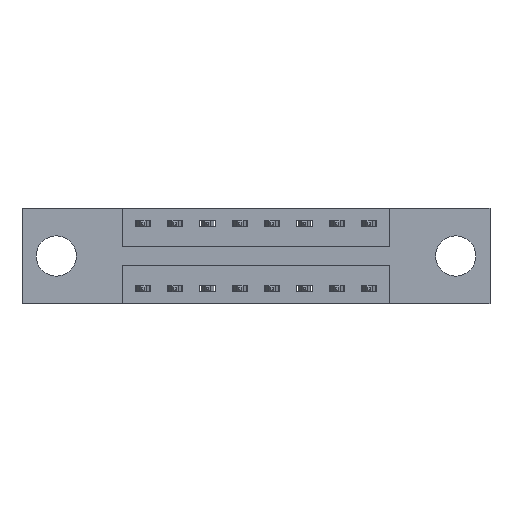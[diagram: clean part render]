
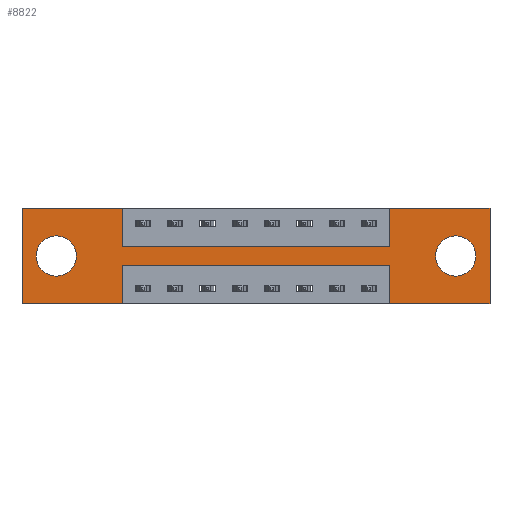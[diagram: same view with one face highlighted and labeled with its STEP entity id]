
A CAD part, front view. The second image highlights one B-rep face of the part: STEP entity #8822.
In plain terms, the highlighted planar face has unit normal (0, -1, 0).
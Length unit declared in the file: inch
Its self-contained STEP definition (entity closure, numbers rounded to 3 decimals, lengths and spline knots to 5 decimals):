
#18 = CIRCLE ( 'NONE', #1250, 0.078 ) ;
#73 = CARTESIAN_POINT ( 'NONE',  ( 0., 0., 0. ) ) ;
#162 = CARTESIAN_POINT ( 'NONE',  ( 0., 0., 0. ) ) ;
#163 = CARTESIAN_POINT ( 'NONE',  ( 1.6775, 0., -0.185 ) ) ;
#220 = CARTESIAN_POINT ( 'NONE',  ( 1.6775, 0., -0.263 ) ) ;
#240 = EDGE_CURVE ( 'NONE', #2358, #2981, #966, .T. ) ;
#244 = ORIENTED_EDGE ( 'NONE', *, *, #4521, .T. ) ;
#248 = VECTOR ( 'NONE', #5914, 39.37008 ) ;
#287 = CARTESIAN_POINT ( 'NONE',  ( 0., 0., -0.37 ) ) ;
#344 = DIRECTION ( 'NONE',  ( -1., 0., 0. ) ) ;
#372 = ORIENTED_EDGE ( 'NONE', *, *, #9281, .T. ) ;
#377 = VECTOR ( 'NONE', #1443, 39.37008 ) ;
#523 = CARTESIAN_POINT ( 'NONE',  ( 0.3875, 0., -0.15 ) ) ;
#602 = VECTOR ( 'NONE', #3147, 39.37008 ) ;
#604 = LINE ( 'NONE', #2105, #8022 ) ;
#612 = EDGE_CURVE ( 'NONE', #4456, #1969, #2550, .T. ) ;
#658 = EDGE_CURVE ( 'NONE', #5437, #5779, #6012, .T. ) ;
#760 = CARTESIAN_POINT ( 'NONE',  ( 0., 0., 0. ) ) ;
#766 = ORIENTED_EDGE ( 'NONE', *, *, #9006, .T. ) ;
#806 = ORIENTED_EDGE ( 'NONE', *, *, #4437, .F. ) ;
#897 = VERTEX_POINT ( 'NONE', #5946 ) ;
#966 = LINE ( 'NONE', #3966, #8792 ) ;
#1250 = AXIS2_PLACEMENT_3D ( 'NONE', #4259, #5805, #4326 ) ;
#1253 = VERTEX_POINT ( 'NONE', #4018 ) ;
#1443 = DIRECTION ( 'NONE',  ( 0., 0., -1. ) ) ;
#1598 = CIRCLE ( 'NONE', #2481, 0.078 ) ;
#1659 = ORIENTED_EDGE ( 'NONE', *, *, #9187, .F. ) ;
#1688 = DIRECTION ( 'NONE',  ( 0., 1., 0. ) ) ;
#1774 = ORIENTED_EDGE ( 'NONE', *, *, #240, .F. ) ;
#1795 = CARTESIAN_POINT ( 'NONE',  ( 0.1325, 0., -0.185 ) ) ;
#1802 = VECTOR ( 'NONE', #2873, 39.37008 ) ;
#1834 = LINE ( 'NONE', #760, #5275 ) ;
#1969 = VERTEX_POINT ( 'NONE', #3968 ) ;
#2040 = CARTESIAN_POINT ( 'NONE',  ( 1.4225, 0., -0.22 ) ) ;
#2066 = FACE_BOUND ( 'NONE', #4221, .T. ) ;
#2105 = CARTESIAN_POINT ( 'NONE',  ( 0., 0., 0. ) ) ;
#2180 = FACE_OUTER_BOUND ( 'NONE', #2342, .T. ) ;
#2183 = CIRCLE ( 'NONE', #5569, 0.078 ) ;
#2309 = FACE_BOUND ( 'NONE', #3071, .T. ) ;
#2311 = VECTOR ( 'NONE', #5316, 39.37008 ) ;
#2342 = EDGE_LOOP ( 'NONE', ( #7362, #7193, #8394, #806, #4942, #7039, #1659, #1774, #8101, #3868, #5143, #7452 ) ) ;
#2358 = VERTEX_POINT ( 'NONE', #523 ) ;
#2362 = VERTEX_POINT ( 'NONE', #7970 ) ;
#2425 = DIRECTION ( 'NONE',  ( 0., -1., 0. ) ) ;
#2481 = AXIS2_PLACEMENT_3D ( 'NONE', #1795, #7072, #8713 ) ;
#2550 = LINE ( 'NONE', #162, #602 ) ;
#2579 = CARTESIAN_POINT ( 'NONE',  ( 0.3875, 0., -0.22 ) ) ;
#2589 = CARTESIAN_POINT ( 'NONE',  ( 0.3875, 0., -0.37 ) ) ;
#2873 = DIRECTION ( 'NONE',  ( -1., 0., 0. ) ) ;
#2916 = EDGE_CURVE ( 'NONE', #5779, #5621, #9279, .T. ) ;
#2950 = VECTOR ( 'NONE', #7378, 39.37008 ) ;
#2981 = VERTEX_POINT ( 'NONE', #9341 ) ;
#2998 = CARTESIAN_POINT ( 'NONE',  ( 1.4225, 0., 0. ) ) ;
#3021 = EDGE_CURVE ( 'NONE', #9406, #4456, #1834, .T. ) ;
#3071 = EDGE_LOOP ( 'NONE', ( #3728, #766 ) ) ;
#3147 = DIRECTION ( 'NONE',  ( 1., 0., 0. ) ) ;
#3158 = DIRECTION ( 'NONE',  ( 0., 1., 0. ) ) ;
#3473 = VECTOR ( 'NONE', #344, 39.37008 ) ;
#3620 = CARTESIAN_POINT ( 'NONE',  ( 0.3875, 0., 0. ) ) ;
#3626 = LINE ( 'NONE', #3620, #377 ) ;
#3728 = ORIENTED_EDGE ( 'NONE', *, *, #3836, .T. ) ;
#3789 = LINE ( 'NONE', #7937, #1802 ) ;
#3836 = EDGE_CURVE ( 'NONE', #2362, #1253, #1598, .T. ) ;
#3864 = LINE ( 'NONE', #5879, #248 ) ;
#3868 = ORIENTED_EDGE ( 'NONE', *, *, #612, .F. ) ;
#3966 = CARTESIAN_POINT ( 'NONE',  ( 0.3875, 0., -0.15 ) ) ;
#3968 = CARTESIAN_POINT ( 'NONE',  ( 0.3875, 0., 0. ) ) ;
#3978 = CARTESIAN_POINT ( 'NONE',  ( 0.3875, 0., -0.37 ) ) ;
#4018 = CARTESIAN_POINT ( 'NONE',  ( 0.1325, 0., -0.263 ) ) ;
#4209 = VECTOR ( 'NONE', #5524, 39.37008 ) ;
#4221 = EDGE_LOOP ( 'NONE', ( #244, #372 ) ) ;
#4259 = CARTESIAN_POINT ( 'NONE',  ( 0.1325, 0., -0.185 ) ) ;
#4326 = DIRECTION ( 'NONE',  ( 0., 0., 1. ) ) ;
#4357 = CARTESIAN_POINT ( 'NONE',  ( 1.6775, 0., -0.107 ) ) ;
#4431 = LINE ( 'NONE', #5045, #2950 ) ;
#4437 = EDGE_CURVE ( 'NONE', #897, #6561, #3864, .T. ) ;
#4456 = VERTEX_POINT ( 'NONE', #73 ) ;
#4521 = EDGE_CURVE ( 'NONE', #7868, #5977, #8732, .T. ) ;
#4560 = VECTOR ( 'NONE', #6499, 39.37008 ) ;
#4563 = AXIS2_PLACEMENT_3D ( 'NONE', #287, #2425, #6246 ) ;
#4712 = CARTESIAN_POINT ( 'NONE',  ( 1.81, 0., 0. ) ) ;
#4804 = CARTESIAN_POINT ( 'NONE',  ( 1.4225, 0., 0. ) ) ;
#4942 = ORIENTED_EDGE ( 'NONE', *, *, #5248, .F. ) ;
#5045 = CARTESIAN_POINT ( 'NONE',  ( 1.4225, 0., -0.37 ) ) ;
#5143 = ORIENTED_EDGE ( 'NONE', *, *, #3021, .F. ) ;
#5198 = DIRECTION ( 'NONE',  ( 1., 0., 0. ) ) ;
#5248 = EDGE_CURVE ( 'NONE', #7309, #897, #6613, .T. ) ;
#5275 = VECTOR ( 'NONE', #7059, 39.37008 ) ;
#5316 = DIRECTION ( 'NONE',  ( 0., 0., 1. ) ) ;
#5411 = VERTEX_POINT ( 'NONE', #4804 ) ;
#5412 = CARTESIAN_POINT ( 'NONE',  ( 0.3875, 0., -0.22 ) ) ;
#5437 = VERTEX_POINT ( 'NONE', #2040 ) ;
#5457 = DIRECTION ( 'NONE',  ( 0., 0., -1. ) ) ;
#5524 = DIRECTION ( 'NONE',  ( 0., 0., -1. ) ) ;
#5569 = AXIS2_PLACEMENT_3D ( 'NONE', #163, #3158, #5457 ) ;
#5621 = VERTEX_POINT ( 'NONE', #2589 ) ;
#5779 = VERTEX_POINT ( 'NONE', #2579 ) ;
#5805 = DIRECTION ( 'NONE',  ( 0., 1., 0. ) ) ;
#5879 = CARTESIAN_POINT ( 'NONE',  ( 0., 0., -0.37 ) ) ;
#5914 = DIRECTION ( 'NONE',  ( -1., 0., 0. ) ) ;
#5946 = CARTESIAN_POINT ( 'NONE',  ( 1.81, 0., -0.37 ) ) ;
#5977 = VERTEX_POINT ( 'NONE', #220 ) ;
#6012 = LINE ( 'NONE', #5412, #3473 ) ;
#6090 = EDGE_CURVE ( 'NONE', #1969, #2358, #3626, .T. ) ;
#6118 = CARTESIAN_POINT ( 'NONE',  ( 1.4225, 0., -0.37 ) ) ;
#6246 = DIRECTION ( 'NONE',  ( 0., 0., -1. ) ) ;
#6499 = DIRECTION ( 'NONE',  ( 0., 0., -1. ) ) ;
#6561 = VERTEX_POINT ( 'NONE', #6118 ) ;
#6613 = LINE ( 'NONE', #4712, #4209 ) ;
#6786 = DIRECTION ( 'NONE',  ( 1., 0., 0. ) ) ;
#7039 = ORIENTED_EDGE ( 'NONE', *, *, #8597, .F. ) ;
#7059 = DIRECTION ( 'NONE',  ( 0., 0., 1. ) ) ;
#7072 = DIRECTION ( 'NONE',  ( 0., 1., 0. ) ) ;
#7193 = ORIENTED_EDGE ( 'NONE', *, *, #658, .F. ) ;
#7254 = EDGE_CURVE ( 'NONE', #6561, #5437, #4431, .T. ) ;
#7309 = VERTEX_POINT ( 'NONE', #8970 ) ;
#7362 = ORIENTED_EDGE ( 'NONE', *, *, #2916, .F. ) ;
#7378 = DIRECTION ( 'NONE',  ( 0., 0., 1. ) ) ;
#7452 = ORIENTED_EDGE ( 'NONE', *, *, #9717, .F. ) ;
#7868 = VERTEX_POINT ( 'NONE', #4357 ) ;
#7937 = CARTESIAN_POINT ( 'NONE',  ( 0., 0., -0.37 ) ) ;
#7970 = CARTESIAN_POINT ( 'NONE',  ( 0.1325, 0., -0.107 ) ) ;
#8022 = VECTOR ( 'NONE', #6786, 39.37008 ) ;
#8101 = ORIENTED_EDGE ( 'NONE', *, *, #6090, .F. ) ;
#8394 = ORIENTED_EDGE ( 'NONE', *, *, #7254, .F. ) ;
#8521 = CARTESIAN_POINT ( 'NONE',  ( 1.6775, 0., -0.185 ) ) ;
#8597 = EDGE_CURVE ( 'NONE', #5411, #7309, #604, .T. ) ;
#8607 = DIRECTION ( 'NONE',  ( 0., 0., -1. ) ) ;
#8713 = DIRECTION ( 'NONE',  ( 0., 0., 1. ) ) ;
#8732 = CIRCLE ( 'NONE', #8815, 0.078 ) ;
#8792 = VECTOR ( 'NONE', #5198, 39.37008 ) ;
#8815 = AXIS2_PLACEMENT_3D ( 'NONE', #8521, #1688, #8607 ) ;
#8822 = ADVANCED_FACE ( 'NONE', ( #2066, #2309, #2180 ), #9411, .T. ) ;
#8970 = CARTESIAN_POINT ( 'NONE',  ( 1.81, 0., 0. ) ) ;
#9006 = EDGE_CURVE ( 'NONE', #1253, #2362, #18, .T. ) ;
#9187 = EDGE_CURVE ( 'NONE', #2981, #5411, #9736, .T. ) ;
#9279 = LINE ( 'NONE', #3978, #4560 ) ;
#9281 = EDGE_CURVE ( 'NONE', #5977, #7868, #2183, .T. ) ;
#9341 = CARTESIAN_POINT ( 'NONE',  ( 1.4225, 0., -0.15 ) ) ;
#9359 = CARTESIAN_POINT ( 'NONE',  ( 0., 0., -0.37 ) ) ;
#9406 = VERTEX_POINT ( 'NONE', #9359 ) ;
#9411 = PLANE ( 'NONE',  #4563 ) ;
#9717 = EDGE_CURVE ( 'NONE', #5621, #9406, #3789, .T. ) ;
#9736 = LINE ( 'NONE', #2998, #2311 ) ;
